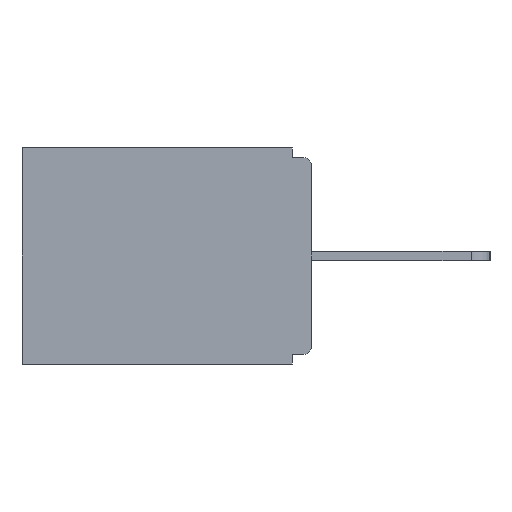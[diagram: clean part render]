
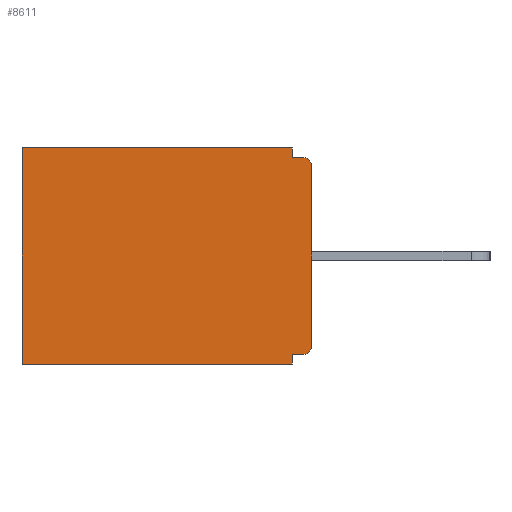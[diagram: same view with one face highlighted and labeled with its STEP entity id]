
A CAD part, left-side view. The second image highlights one B-rep face of the part: STEP entity #8611.
In plain terms, the highlighted planar face has unit normal (-1, 0, 0).
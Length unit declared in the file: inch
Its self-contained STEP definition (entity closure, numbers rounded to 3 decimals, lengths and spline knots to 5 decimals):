
#225 = VERTEX_POINT ( 'NONE', #14873 ) ;
#258 = VECTOR ( 'NONE', #2131, 39.37008 ) ;
#395 = VERTEX_POINT ( 'NONE', #1220 ) ;
#528 = EDGE_CURVE ( 'NONE', #5432, #2781, #14988, .T. ) ;
#738 = LINE ( 'NONE', #5532, #19821 ) ;
#1220 = CARTESIAN_POINT ( 'NONE',  ( 0.298, 0.031, 0. ) ) ;
#1368 = ORIENTED_EDGE ( 'NONE', *, *, #12569, .T. ) ;
#1395 = VERTEX_POINT ( 'NONE', #2173 ) ;
#1651 = DIRECTION ( 'NONE',  ( 0., 0., -1. ) ) ;
#2020 = ORIENTED_EDGE ( 'NONE', *, *, #9809, .T. ) ;
#2108 = CARTESIAN_POINT ( 'NONE',  ( 0.298, 0., 0. ) ) ;
#2131 = DIRECTION ( 'NONE',  ( 0., 0., -1. ) ) ;
#2173 = CARTESIAN_POINT ( 'NONE',  ( 0.298, 0.46, 0. ) ) ;
#2175 = VECTOR ( 'NONE', #16083, 39.37008 ) ;
#2183 = VECTOR ( 'NONE', #11998, 39.37008 ) ;
#2211 = ORIENTED_EDGE ( 'NONE', *, *, #10430, .F. ) ;
#2653 = ORIENTED_EDGE ( 'NONE', *, *, #17196, .F. ) ;
#2781 = VERTEX_POINT ( 'NONE', #11260 ) ;
#3364 = VERTEX_POINT ( 'NONE', #12538 ) ;
#3445 = VECTOR ( 'NONE', #23633, 39.37008 ) ;
#3785 = DIRECTION ( 'NONE',  ( -1., 0., 0. ) ) ;
#3829 = ORIENTED_EDGE ( 'NONE', *, *, #22813, .F. ) ;
#3833 = ORIENTED_EDGE ( 'NONE', *, *, #528, .F. ) ;
#4201 = EDGE_CURVE ( 'NONE', #395, #1395, #8352, .T. ) ;
#4674 = CARTESIAN_POINT ( 'NONE',  ( 0.298, 0.46, 0. ) ) ;
#4823 = AXIS2_PLACEMENT_3D ( 'NONE', #23546, #12794, #1651 ) ;
#5000 = CIRCLE ( 'NONE', #4823, 0.015 ) ;
#5377 = LINE ( 'NONE', #2108, #258 ) ;
#5432 = VERTEX_POINT ( 'NONE', #16660 ) ;
#5532 = CARTESIAN_POINT ( 'NONE',  ( 0.298, 0.031, -0.343 ) ) ;
#6384 = VECTOR ( 'NONE', #9493, 39.37008 ) ;
#6619 = AXIS2_PLACEMENT_3D ( 'NONE', #14237, #6971, #19760 ) ;
#6883 = EDGE_CURVE ( 'NONE', #22162, #3364, #5377, .T. ) ;
#6971 = DIRECTION ( 'NONE',  ( 1., 0., 0. ) ) ;
#7436 = VERTEX_POINT ( 'NONE', #11959 ) ;
#7740 = LINE ( 'NONE', #4674, #2183 ) ;
#8352 = LINE ( 'NONE', #16969, #3445 ) ;
#8611 = ADVANCED_FACE ( 'NONE', ( #17973 ), #8757, .F. ) ;
#8757 = PLANE ( 'NONE',  #6619 ) ;
#8870 = DIRECTION ( 'NONE',  ( 0., 0., -1. ) ) ;
#9336 = EDGE_LOOP ( 'NONE', ( #2020, #2653, #11808, #21322, #1368, #3829, #2211, #3833, #21098, #23216 ) ) ;
#9410 = CARTESIAN_POINT ( 'NONE',  ( 0.298, 0., -0.015 ) ) ;
#9493 = DIRECTION ( 'NONE',  ( 0., -1., 0. ) ) ;
#9502 = VECTOR ( 'NONE', #11787, 39.37008 ) ;
#9611 = LINE ( 'NONE', #12576, #15095 ) ;
#9809 = EDGE_CURVE ( 'NONE', #22162, #19804, #5000, .T. ) ;
#10430 = EDGE_CURVE ( 'NONE', #2781, #12387, #738, .T. ) ;
#11260 = CARTESIAN_POINT ( 'NONE',  ( 0.298, 0.031, -0.328 ) ) ;
#11787 = DIRECTION ( 'NONE',  ( 0., 1., 0. ) ) ;
#11808 = ORIENTED_EDGE ( 'NONE', *, *, #15356, .F. ) ;
#11959 = CARTESIAN_POINT ( 'NONE',  ( 0.298, 0.031, -0.015 ) ) ;
#11998 = DIRECTION ( 'NONE',  ( 0., 0., -1. ) ) ;
#12307 = EDGE_CURVE ( 'NONE', #5432, #3364, #13772, .T. ) ;
#12387 = VERTEX_POINT ( 'NONE', #22292 ) ;
#12538 = CARTESIAN_POINT ( 'NONE',  ( 0.298, 0., -0.313 ) ) ;
#12569 = EDGE_CURVE ( 'NONE', #1395, #225, #7740, .T. ) ;
#12576 = CARTESIAN_POINT ( 'NONE',  ( 0.298, 0.031, -0.343 ) ) ;
#12639 = LINE ( 'NONE', #23235, #2175 ) ;
#12794 = DIRECTION ( 'NONE',  ( -1., 0., 0. ) ) ;
#13772 = CIRCLE ( 'NONE', #13786, 0.015 ) ;
#13786 = AXIS2_PLACEMENT_3D ( 'NONE', #14816, #3785, #16628 ) ;
#13837 = CARTESIAN_POINT ( 'NONE',  ( 0.298, 0., -0.328 ) ) ;
#14237 = CARTESIAN_POINT ( 'NONE',  ( 0.298, 0., 0. ) ) ;
#14816 = CARTESIAN_POINT ( 'NONE',  ( 0.298, 0.015, -0.313 ) ) ;
#14873 = CARTESIAN_POINT ( 'NONE',  ( 0.298, 0.46, -0.343 ) ) ;
#14988 = LINE ( 'NONE', #13837, #9502 ) ;
#15095 = VECTOR ( 'NONE', #8870, 39.37008 ) ;
#15356 = EDGE_CURVE ( 'NONE', #395, #7436, #9611, .T. ) ;
#16083 = DIRECTION ( 'NONE',  ( 0., 1., 0. ) ) ;
#16172 = LINE ( 'NONE', #9410, #6384 ) ;
#16628 = DIRECTION ( 'NONE',  ( 0., 0., -1. ) ) ;
#16660 = CARTESIAN_POINT ( 'NONE',  ( 0.298, 0.015, -0.328 ) ) ;
#16969 = CARTESIAN_POINT ( 'NONE',  ( 0.298, 0., 0. ) ) ;
#17196 = EDGE_CURVE ( 'NONE', #7436, #19804, #16172, .T. ) ;
#17973 = FACE_OUTER_BOUND ( 'NONE', #9336, .T. ) ;
#18154 = CARTESIAN_POINT ( 'NONE',  ( 0.298, 0., -0.03 ) ) ;
#18331 = DIRECTION ( 'NONE',  ( 0., 0., -1. ) ) ;
#19760 = DIRECTION ( 'NONE',  ( 0., 0., -1. ) ) ;
#19804 = VERTEX_POINT ( 'NONE', #20314 ) ;
#19821 = VECTOR ( 'NONE', #18331, 39.37008 ) ;
#20314 = CARTESIAN_POINT ( 'NONE',  ( 0.298, 0.015, -0.015 ) ) ;
#21098 = ORIENTED_EDGE ( 'NONE', *, *, #12307, .T. ) ;
#21322 = ORIENTED_EDGE ( 'NONE', *, *, #4201, .T. ) ;
#22162 = VERTEX_POINT ( 'NONE', #18154 ) ;
#22292 = CARTESIAN_POINT ( 'NONE',  ( 0.298, 0.031, -0.343 ) ) ;
#22813 = EDGE_CURVE ( 'NONE', #12387, #225, #12639, .T. ) ;
#23216 = ORIENTED_EDGE ( 'NONE', *, *, #6883, .F. ) ;
#23235 = CARTESIAN_POINT ( 'NONE',  ( 0.298, 0., -0.343 ) ) ;
#23546 = CARTESIAN_POINT ( 'NONE',  ( 0.298, 0.015, -0.03 ) ) ;
#23633 = DIRECTION ( 'NONE',  ( 0., 1., 0. ) ) ;
